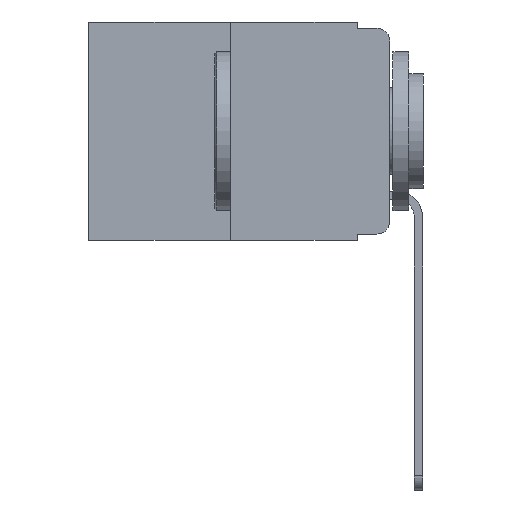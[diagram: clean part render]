
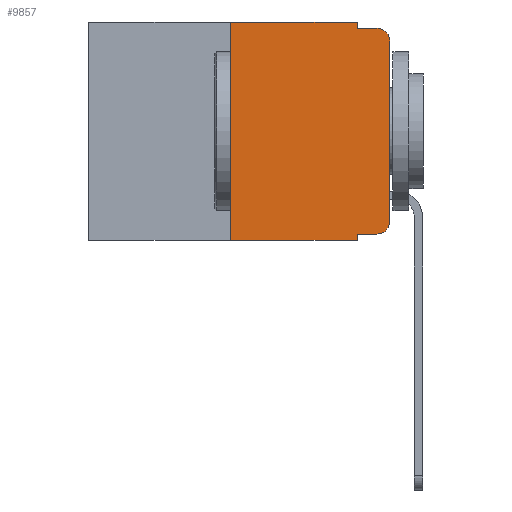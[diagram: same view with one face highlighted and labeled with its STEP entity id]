
A CAD part, left-side view. The second image highlights one B-rep face of the part: STEP entity #9857.
In plain terms, the highlighted planar face has unit normal (-1, 0, 0).
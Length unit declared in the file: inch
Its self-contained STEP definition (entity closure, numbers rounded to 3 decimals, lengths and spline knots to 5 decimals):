
#111 = VERTEX_POINT ( 'NONE', #552 ) ;
#248 = DIRECTION ( 'NONE',  ( 0., 0., -1. ) ) ;
#308 = EDGE_CURVE ( 'NONE', #5235, #8747, #606, .T. ) ;
#399 = ORIENTED_EDGE ( 'NONE', *, *, #5152, .T. ) ;
#503 = DIRECTION ( 'NONE',  ( 0., 0., -1. ) ) ;
#552 = CARTESIAN_POINT ( 'NONE',  ( 0., 0.051, 0. ) ) ;
#598 = VERTEX_POINT ( 'NONE', #8418 ) ;
#606 = LINE ( 'NONE', #10676, #9152 ) ;
#640 = LINE ( 'NONE', #9153, #8851 ) ;
#728 = VERTEX_POINT ( 'NONE', #1071 ) ;
#1071 = CARTESIAN_POINT ( 'NONE',  ( 0., 0., -0.313 ) ) ;
#1226 = ORIENTED_EDGE ( 'NONE', *, *, #308, .T. ) ;
#1287 = PLANE ( 'NONE',  #10582 ) ;
#1940 = VECTOR ( 'NONE', #11158, 39.37008 ) ;
#1989 = CARTESIAN_POINT ( 'NONE',  ( 0., 0., -0.03 ) ) ;
#2079 = ORIENTED_EDGE ( 'NONE', *, *, #13457, .F. ) ;
#2282 = EDGE_CURVE ( 'NONE', #728, #8889, #8114, .T. ) ;
#2334 = CARTESIAN_POINT ( 'NONE',  ( 0., 0.473, 0. ) ) ;
#2379 = DIRECTION ( 'NONE',  ( 0., 0., -1. ) ) ;
#2655 = EDGE_CURVE ( 'NONE', #8770, #13516, #640, .T. ) ;
#2901 = DIRECTION ( 'NONE',  ( 0., 0., 1. ) ) ;
#3024 = DIRECTION ( 'NONE',  ( 0., -1., 0. ) ) ;
#3500 = LINE ( 'NONE', #9299, #5895 ) ;
#3709 = EDGE_CURVE ( 'NONE', #111, #7000, #8838, .T. ) ;
#4121 = ORIENTED_EDGE ( 'NONE', *, *, #3709, .F. ) ;
#4816 = CARTESIAN_POINT ( 'NONE',  ( 0., 0.051, 0. ) ) ;
#4880 = DIRECTION ( 'NONE',  ( -1., 0., 0. ) ) ;
#4914 = CARTESIAN_POINT ( 'NONE',  ( 0., 0.02, -0.333 ) ) ;
#5091 = ORIENTED_EDGE ( 'NONE', *, *, #6988, .F. ) ;
#5152 = EDGE_CURVE ( 'NONE', #8889, #598, #8468, .T. ) ;
#5235 = VERTEX_POINT ( 'NONE', #9600 ) ;
#5321 = DIRECTION ( 'NONE',  ( -1., 0., 0. ) ) ;
#5377 = VECTOR ( 'NONE', #503, 39.37008 ) ;
#5514 = FACE_OUTER_BOUND ( 'NONE', #7778, .T. ) ;
#5895 = VECTOR ( 'NONE', #3024, 39.37008 ) ;
#5969 = ORIENTED_EDGE ( 'NONE', *, *, #13556, .F. ) ;
#6384 = AXIS2_PLACEMENT_3D ( 'NONE', #11131, #4880, #12128 ) ;
#6988 = EDGE_CURVE ( 'NONE', #10398, #111, #3500, .T. ) ;
#7000 = VERTEX_POINT ( 'NONE', #13339 ) ;
#7007 = CARTESIAN_POINT ( 'NONE',  ( 0., 0.051, -0.343 ) ) ;
#7528 = LINE ( 'NONE', #8133, #12619 ) ;
#7778 = EDGE_LOOP ( 'NONE', ( #9143, #399, #5969, #4121, #5091, #8840, #12459, #2079, #1226, #9193 ) ) ;
#8114 = LINE ( 'NONE', #8680, #13500 ) ;
#8133 = CARTESIAN_POINT ( 'NONE',  ( 0., 0.25, 0. ) ) ;
#8418 = CARTESIAN_POINT ( 'NONE',  ( 0., 0.02, -0.01 ) ) ;
#8468 = CIRCLE ( 'NONE', #13718, 0.02 ) ;
#8680 = CARTESIAN_POINT ( 'NONE',  ( 0., 0., 0. ) ) ;
#8697 = DIRECTION ( 'NONE',  ( 1., 0., 0. ) ) ;
#8747 = VERTEX_POINT ( 'NONE', #4914 ) ;
#8770 = VERTEX_POINT ( 'NONE', #9189 ) ;
#8838 = LINE ( 'NONE', #9557, #11215 ) ;
#8840 = ORIENTED_EDGE ( 'NONE', *, *, #10180, .F. ) ;
#8851 = VECTOR ( 'NONE', #11474, 39.37008 ) ;
#8889 = VERTEX_POINT ( 'NONE', #1989 ) ;
#9143 = ORIENTED_EDGE ( 'NONE', *, *, #2282, .T. ) ;
#9148 = DIRECTION ( 'NONE',  ( 0., 0., 1. ) ) ;
#9152 = VECTOR ( 'NONE', #10357, 39.37008 ) ;
#9153 = CARTESIAN_POINT ( 'NONE',  ( 0., 0.473, -0.343 ) ) ;
#9189 = CARTESIAN_POINT ( 'NONE',  ( 0., 0.25, -0.343 ) ) ;
#9193 = ORIENTED_EDGE ( 'NONE', *, *, #12783, .T. ) ;
#9299 = CARTESIAN_POINT ( 'NONE',  ( 0., 0.473, 0. ) ) ;
#9557 = CARTESIAN_POINT ( 'NONE',  ( 0., 0.051, 0. ) ) ;
#9600 = CARTESIAN_POINT ( 'NONE',  ( 0., 0.051, -0.333 ) ) ;
#9857 = ADVANCED_FACE ( 'NONE', ( #5514 ), #1287, .F. ) ;
#10153 = CIRCLE ( 'NONE', #6384, 0.02 ) ;
#10180 = EDGE_CURVE ( 'NONE', #8770, #10398, #7528, .T. ) ;
#10357 = DIRECTION ( 'NONE',  ( 0., -1., 0. ) ) ;
#10398 = VERTEX_POINT ( 'NONE', #13491 ) ;
#10582 = AXIS2_PLACEMENT_3D ( 'NONE', #2334, #8697, #2379 ) ;
#10676 = CARTESIAN_POINT ( 'NONE',  ( 0., 0.051, -0.333 ) ) ;
#10940 = LINE ( 'NONE', #13216, #1940 ) ;
#11131 = CARTESIAN_POINT ( 'NONE',  ( 0., 0.02, -0.313 ) ) ;
#11158 = DIRECTION ( 'NONE',  ( 0., -1., 0. ) ) ;
#11215 = VECTOR ( 'NONE', #248, 39.37008 ) ;
#11474 = DIRECTION ( 'NONE',  ( 0., -1., 0. ) ) ;
#11548 = CARTESIAN_POINT ( 'NONE',  ( 0., 0.02, -0.03 ) ) ;
#12128 = DIRECTION ( 'NONE',  ( 0., 0., -1. ) ) ;
#12459 = ORIENTED_EDGE ( 'NONE', *, *, #2655, .T. ) ;
#12538 = DIRECTION ( 'NONE',  ( 0., 0., -1. ) ) ;
#12619 = VECTOR ( 'NONE', #2901, 39.37008 ) ;
#12783 = EDGE_CURVE ( 'NONE', #8747, #728, #10153, .T. ) ;
#13216 = CARTESIAN_POINT ( 'NONE',  ( 0., 0.051, -0.01 ) ) ;
#13339 = CARTESIAN_POINT ( 'NONE',  ( 0., 0.051, -0.01 ) ) ;
#13457 = EDGE_CURVE ( 'NONE', #5235, #13516, #13607, .T. ) ;
#13491 = CARTESIAN_POINT ( 'NONE',  ( 0., 0.25, 0. ) ) ;
#13500 = VECTOR ( 'NONE', #9148, 39.37008 ) ;
#13516 = VERTEX_POINT ( 'NONE', #7007 ) ;
#13556 = EDGE_CURVE ( 'NONE', #7000, #598, #10940, .T. ) ;
#13607 = LINE ( 'NONE', #4816, #5377 ) ;
#13718 = AXIS2_PLACEMENT_3D ( 'NONE', #11548, #5321, #12538 ) ;
